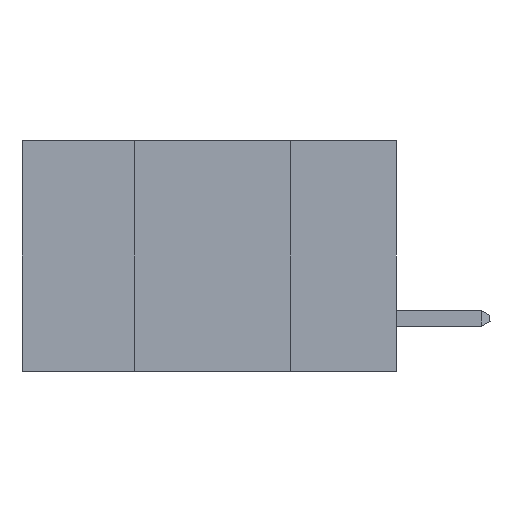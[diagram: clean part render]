
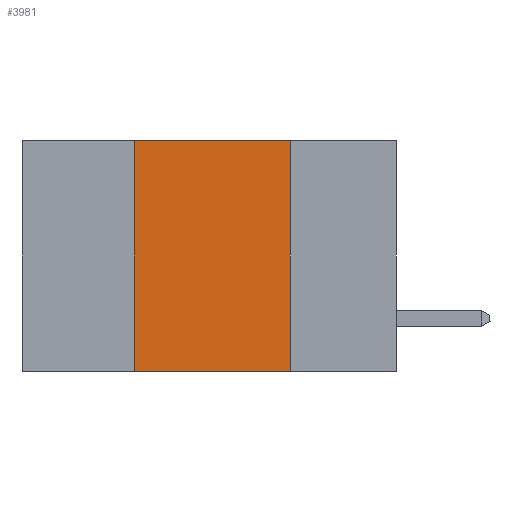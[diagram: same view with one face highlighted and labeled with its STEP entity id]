
A CAD part, left-side view. The second image highlights one B-rep face of the part: STEP entity #3981.
In plain terms, the highlighted planar face has unit normal (-1, 0, 0).
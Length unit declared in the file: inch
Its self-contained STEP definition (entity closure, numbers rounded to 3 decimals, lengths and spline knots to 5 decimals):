
#931 = EDGE_LOOP ( 'NONE', ( #4941, #13856, #15241, #3042 ) ) ;
#1291 = CARTESIAN_POINT ( 'NONE',  ( 0., 0.6, 0. ) ) ;
#1620 = FACE_OUTER_BOUND ( 'NONE', #931, .T. ) ;
#1754 = VERTEX_POINT ( 'NONE', #12843 ) ;
#2084 = VECTOR ( 'NONE', #8302, 39.37008 ) ;
#2779 = CARTESIAN_POINT ( 'NONE',  ( 0., 0.42, 0. ) ) ;
#2911 = LINE ( 'NONE', #15539, #10133 ) ;
#3042 = ORIENTED_EDGE ( 'NONE', *, *, #14299, .T. ) ;
#3720 = LINE ( 'NONE', #3769, #11794 ) ;
#3769 = CARTESIAN_POINT ( 'NONE',  ( 0., 0.6, -0.37 ) ) ;
#3981 = ADVANCED_FACE ( 'NONE', ( #1620 ), #6452, .F. ) ;
#4072 = CARTESIAN_POINT ( 'NONE',  ( 0., 0.6, 0. ) ) ;
#4941 = ORIENTED_EDGE ( 'NONE', *, *, #7464, .F. ) ;
#6452 = PLANE ( 'NONE',  #10795 ) ;
#6932 = CARTESIAN_POINT ( 'NONE',  ( 0., 0.42, -0.37 ) ) ;
#7464 = EDGE_CURVE ( 'NONE', #1754, #10674, #2911, .T. ) ;
#7507 = CARTESIAN_POINT ( 'NONE',  ( 0., 0.17, -0.37 ) ) ;
#8302 = DIRECTION ( 'NONE',  ( 0., -1., 0. ) ) ;
#8340 = LINE ( 'NONE', #4072, #2084 ) ;
#9124 = DIRECTION ( 'NONE',  ( 0., -1., 0. ) ) ;
#9861 = EDGE_CURVE ( 'NONE', #13465, #1754, #8340, .T. ) ;
#10133 = VECTOR ( 'NONE', #15769, 39.37008 ) ;
#10674 = VERTEX_POINT ( 'NONE', #7507 ) ;
#10795 = AXIS2_PLACEMENT_3D ( 'NONE', #1291, #15320, #15531 ) ;
#11794 = VECTOR ( 'NONE', #9124, 39.37008 ) ;
#12486 = VERTEX_POINT ( 'NONE', #6932 ) ;
#12843 = CARTESIAN_POINT ( 'NONE',  ( 0., 0.17, 0. ) ) ;
#13465 = VERTEX_POINT ( 'NONE', #15360 ) ;
#13856 = ORIENTED_EDGE ( 'NONE', *, *, #9861, .F. ) ;
#14299 = EDGE_CURVE ( 'NONE', #12486, #10674, #3720, .T. ) ;
#14759 = EDGE_CURVE ( 'NONE', #12486, #13465, #16355, .T. ) ;
#15241 = ORIENTED_EDGE ( 'NONE', *, *, #14759, .F. ) ;
#15320 = DIRECTION ( 'NONE',  ( 1., 0., 0. ) ) ;
#15344 = DIRECTION ( 'NONE',  ( 0., 0., 1. ) ) ;
#15360 = CARTESIAN_POINT ( 'NONE',  ( 0., 0.42, 0. ) ) ;
#15531 = DIRECTION ( 'NONE',  ( 0., 0., -1. ) ) ;
#15539 = CARTESIAN_POINT ( 'NONE',  ( 0., 0.17, 0. ) ) ;
#15556 = VECTOR ( 'NONE', #15344, 39.37008 ) ;
#15769 = DIRECTION ( 'NONE',  ( 0., 0., -1. ) ) ;
#16355 = LINE ( 'NONE', #2779, #15556 ) ;
